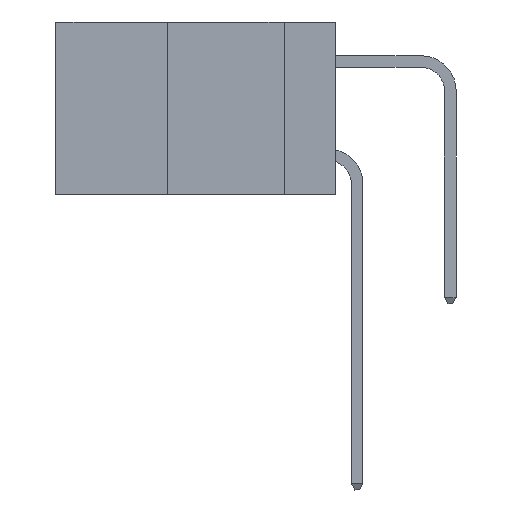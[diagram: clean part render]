
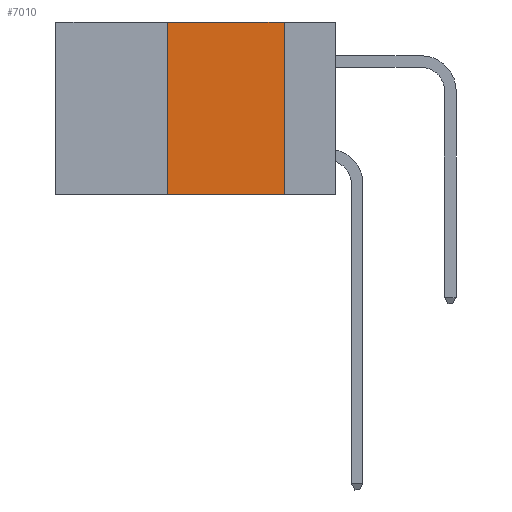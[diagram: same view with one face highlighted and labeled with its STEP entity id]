
A CAD part, left-side view. The second image highlights one B-rep face of the part: STEP entity #7010.
In plain terms, the highlighted planar face has unit normal (-1, 0, 0).
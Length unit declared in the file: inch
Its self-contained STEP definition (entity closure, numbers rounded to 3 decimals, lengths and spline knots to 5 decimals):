
#1259 = CARTESIAN_POINT ( 'NONE',  ( 0., 0.36, -0.37 ) ) ;
#1593 = VECTOR ( 'NONE', #14611, 39.37008 ) ;
#1961 = LINE ( 'NONE', #7403, #6700 ) ;
#2080 = ORIENTED_EDGE ( 'NONE', *, *, #14067, .T. ) ;
#2165 = VERTEX_POINT ( 'NONE', #1259 ) ;
#2290 = DIRECTION ( 'NONE',  ( 0., 0., -1. ) ) ;
#2409 = ORIENTED_EDGE ( 'NONE', *, *, #13494, .F. ) ;
#2726 = EDGE_CURVE ( 'NONE', #3086, #6319, #10881, .T. ) ;
#2794 = CARTESIAN_POINT ( 'NONE',  ( 0., 0.11, 0. ) ) ;
#2829 = DIRECTION ( 'NONE',  ( 0., 0., -1. ) ) ;
#3086 = VERTEX_POINT ( 'NONE', #2794 ) ;
#3540 = FACE_OUTER_BOUND ( 'NONE', #9196, .T. ) ;
#3555 = DIRECTION ( 'NONE',  ( 0., 0., 1. ) ) ;
#4933 = VECTOR ( 'NONE', #2829, 39.37008 ) ;
#5298 = ORIENTED_EDGE ( 'NONE', *, *, #17092, .F. ) ;
#6319 = VERTEX_POINT ( 'NONE', #11695 ) ;
#6549 = ORIENTED_EDGE ( 'NONE', *, *, #2726, .F. ) ;
#6700 = VECTOR ( 'NONE', #3555, 39.37008 ) ;
#7010 = ADVANCED_FACE ( 'NONE', ( #3540 ), #8999, .F. ) ;
#7403 = CARTESIAN_POINT ( 'NONE',  ( 0., 0.36, 0. ) ) ;
#7650 = CARTESIAN_POINT ( 'NONE',  ( 0., 0.6, -0.37 ) ) ;
#7734 = LINE ( 'NONE', #7650, #1593 ) ;
#8322 = DIRECTION ( 'NONE',  ( 0., -1., 0. ) ) ;
#8785 = VECTOR ( 'NONE', #8322, 39.37008 ) ;
#8999 = PLANE ( 'NONE',  #11156 ) ;
#9196 = EDGE_LOOP ( 'NONE', ( #6549, #5298, #2409, #2080 ) ) ;
#10881 = LINE ( 'NONE', #12226, #4933 ) ;
#11156 = AXIS2_PLACEMENT_3D ( 'NONE', #14446, #11864, #2290 ) ;
#11695 = CARTESIAN_POINT ( 'NONE',  ( 0., 0.11, -0.37 ) ) ;
#11864 = DIRECTION ( 'NONE',  ( 1., 0., 0. ) ) ;
#12226 = CARTESIAN_POINT ( 'NONE',  ( 0., 0.11, 0. ) ) ;
#12446 = CARTESIAN_POINT ( 'NONE',  ( 0., 0.6, 0. ) ) ;
#13408 = CARTESIAN_POINT ( 'NONE',  ( 0., 0.36, 0. ) ) ;
#13494 = EDGE_CURVE ( 'NONE', #2165, #14636, #1961, .T. ) ;
#14067 = EDGE_CURVE ( 'NONE', #2165, #6319, #7734, .T. ) ;
#14446 = CARTESIAN_POINT ( 'NONE',  ( 0., 0.6, 0. ) ) ;
#14611 = DIRECTION ( 'NONE',  ( 0., -1., 0. ) ) ;
#14636 = VERTEX_POINT ( 'NONE', #13408 ) ;
#16714 = LINE ( 'NONE', #12446, #8785 ) ;
#17092 = EDGE_CURVE ( 'NONE', #14636, #3086, #16714, .T. ) ;
